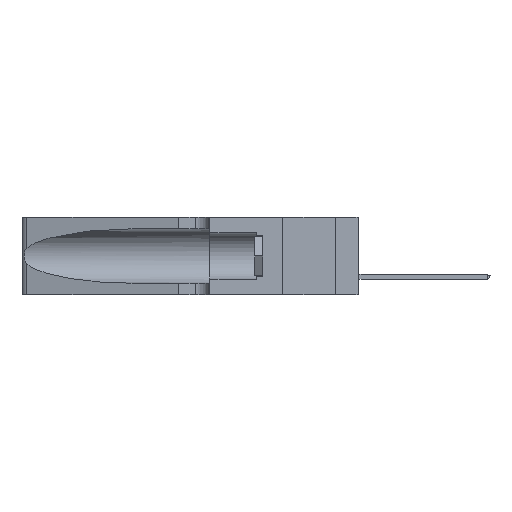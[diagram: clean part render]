
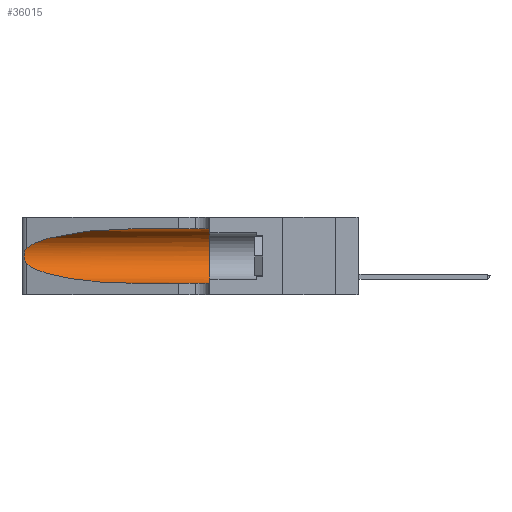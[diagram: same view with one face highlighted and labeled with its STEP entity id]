
A CAD part, left-side view. The second image highlights one B-rep face of the part: STEP entity #36015.
In plain terms, the highlighted cylindrical face has radius 3.308 mm (diameter 6.617 mm), a partial arc.
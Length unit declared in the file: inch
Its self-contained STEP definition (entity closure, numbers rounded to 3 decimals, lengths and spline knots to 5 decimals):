
#264 = CARTESIAN_POINT ( 'NONE',  ( 0.26075, 1.23896, 0.178 ) ) ;
#397 = CARTESIAN_POINT ( 'NONE',  ( 0.25487, 1.22718, 0.14631 ) ) ;
#412 = FACE_OUTER_BOUND ( 'NONE', #27075, .T. ) ;
#540 = CARTESIAN_POINT ( 'NONE',  ( 0.2373, 1.15595, 0.08982 ) ) ;
#809 = EDGE_CURVE ( 'NONE', #25328, #8005, #32476, .T. ) ;
#1909 = DIRECTION ( 'NONE',  ( 0., -1., 0. ) ) ;
#2008 = CYLINDRICAL_SURFACE ( 'NONE', #19978, 0.13025 ) ;
#3634 = CARTESIAN_POINT ( 'NONE',  ( 0.25789, 1.23486, 0.15765 ) ) ;
#3771 = CARTESIAN_POINT ( 'NONE',  ( 0.25555, 1.22993, 0.14849 ) ) ;
#4053 = CARTESIAN_POINT ( 'NONE',  ( 0.1305, 0.72297, 0.05475 ) ) ;
#4175 =( BOUNDED_CURVE ( )  B_SPLINE_CURVE ( 3, ( #26989, #540, #23588, #4053 ),
 .UNSPECIFIED., .F., .F. ) 
 B_SPLINE_CURVE_WITH_KNOTS ( ( 4, 4 ),
 ( 3.44316, 4.71239 ),
 .UNSPECIFIED. ) 
 CURVE ( )  GEOMETRIC_REPRESENTATION_ITEM ( )  RATIONAL_B_SPLINE_CURVE ( ( 1., 0.87, 0.87, 1. ) ) 
 REPRESENTATION_ITEM ( '' )  );
#4190 = CARTESIAN_POINT ( 'NONE',  ( 0.1305, 1.61858, 0.185 ) ) ;
#5490 = VERTEX_POINT ( 'NONE', #7061 ) ;
#6011 = ORIENTED_EDGE ( 'NONE', *, *, #38743, .T. ) ;
#6385 = EDGE_CURVE ( 'NONE', #8803, #22679, #4175, .T. ) ;
#6594 = EDGE_CURVE ( 'NONE', #8005, #26470, #9906, .T. ) ;
#7061 = CARTESIAN_POINT ( 'NONE',  ( 0.25487, 1.22718, 0.22369 ) ) ;
#7087 = CARTESIAN_POINT ( 'NONE',  ( 0.26075, 1.23896, 0.19203 ) ) ;
#8005 = VERTEX_POINT ( 'NONE', #24987 ) ;
#8803 = VERTEX_POINT ( 'NONE', #29382 ) ;
#9710 = ORIENTED_EDGE ( 'NONE', *, *, #809, .F. ) ;
#9906 = CIRCLE ( 'NONE', #33426, 0.13025 ) ;
#10192 = CARTESIAN_POINT ( 'NONE',  ( 0.25487, 1.22718, 0.22369 ) ) ;
#10298 = ORIENTED_EDGE ( 'NONE', *, *, #27484, .T. ) ;
#10596 = CARTESIAN_POINT ( 'NONE',  ( 0.26017, 1.23833, 0.17102 ) ) ;
#12334 = CARTESIAN_POINT ( 'NONE',  ( 0.18966, 0.96281, 0.31525 ) ) ;
#12624 = CARTESIAN_POINT ( 'NONE',  ( 0.25487, 1.22718, 0.22369 ) ) ;
#13598 = VECTOR ( 'NONE', #14438, 39.37008 ) ;
#13793 = CARTESIAN_POINT ( 'NONE',  ( 0.25555, 1.22994, 0.2215 ) ) ;
#13797 = DIRECTION ( 'NONE',  ( 0., -1., 0. ) ) ;
#14438 = DIRECTION ( 'NONE',  ( 0., -1., 0. ) ) ;
#15375 = LINE ( 'NONE', #21896, #42030 ) ;
#15705 = CARTESIAN_POINT ( 'NONE',  ( 0.2373, 1.15595, 0.28018 ) ) ;
#16502 = CARTESIAN_POINT ( 'NONE',  ( 0.1305, 0.72297, 0.05475 ) ) ;
#16868 = CARTESIAN_POINT ( 'NONE',  ( 0.26018, 1.23835, 0.19895 ) ) ;
#17226 =( BOUNDED_CURVE ( )  B_SPLINE_CURVE ( 3, ( #35673, #12334, #15705, #12624 ),
 .UNSPECIFIED., .F., .T. ) 
 B_SPLINE_CURVE_WITH_KNOTS ( ( 4, 4 ),
 ( 1.5708, 2.84003 ),
 .UNSPECIFIED. ) 
 CURVE ( )  GEOMETRIC_REPRESENTATION_ITEM ( )  RATIONAL_B_SPLINE_CURVE ( ( 1., 0.87, 0.87, 1. ) ) 
 REPRESENTATION_ITEM ( '' )  );
#17642 = CARTESIAN_POINT ( 'NONE',  ( 0.1305, 1.61858, 0.31525 ) ) ;
#19507 = ORIENTED_EDGE ( 'NONE', *, *, #6385, .T. ) ;
#19978 = AXIS2_PLACEMENT_3D ( 'NONE', #4190, #13797, #37297 ) ;
#21734 = DIRECTION ( 'NONE',  ( 0., 0., 1. ) ) ;
#21896 = CARTESIAN_POINT ( 'NONE',  ( 0.1305, 1.61858, 0.05475 ) ) ;
#22679 = VERTEX_POINT ( 'NONE', #16502 ) ;
#23378 = EDGE_CURVE ( 'NONE', #22679, #26470, #15375, .T. ) ;
#23588 = CARTESIAN_POINT ( 'NONE',  ( 0.18966, 0.96281, 0.05475 ) ) ;
#24987 = CARTESIAN_POINT ( 'NONE',  ( 0.1305, 0.35, 0.31525 ) ) ;
#25328 = VERTEX_POINT ( 'NONE', #25756 ) ;
#25348 = ORIENTED_EDGE ( 'NONE', *, *, #23378, .T. ) ;
#25756 = CARTESIAN_POINT ( 'NONE',  ( 0.1305, 0.72297, 0.31525 ) ) ;
#26470 = VERTEX_POINT ( 'NONE', #28781 ) ;
#26989 = CARTESIAN_POINT ( 'NONE',  ( 0.25487, 1.22718, 0.14631 ) ) ;
#27075 = EDGE_LOOP ( 'NONE', ( #6011, #10298, #19507, #25348, #29213, #9710 ) ) ;
#27132 = CARTESIAN_POINT ( 'NONE',  ( 0.25639, 1.23184, 0.21858 ) ) ;
#27484 = EDGE_CURVE ( 'NONE', #5490, #8803, #28827, .T. ) ;
#28288 = CARTESIAN_POINT ( 'NONE',  ( 0.1305, 0.35, 0.185 ) ) ;
#28781 = CARTESIAN_POINT ( 'NONE',  ( 0.1305, 0.35, 0.05475 ) ) ;
#28827 = B_SPLINE_CURVE_WITH_KNOTS ( 'NONE', 3,
 ( #10192, #13793, #27132, #37142, #30620, #16868, #7087, #264, #10596, #40218, #3634, #37000, #3771, #397 ),
 .UNSPECIFIED., .F., .F.,
 ( 4, 2, 2, 2, 2, 2, 4 ),
 ( 0., 0.00027, 0.00053, 0.00107, 0.0016, 0.00187, 0.00214 ),
 .UNSPECIFIED. ) ;
#29213 = ORIENTED_EDGE ( 'NONE', *, *, #6594, .F. ) ;
#29382 = CARTESIAN_POINT ( 'NONE',  ( 0.25487, 1.22718, 0.14631 ) ) ;
#30620 = CARTESIAN_POINT ( 'NONE',  ( 0.25854, 1.2359, 0.20912 ) ) ;
#32476 = LINE ( 'NONE', #17642, #13598 ) ;
#33426 = AXIS2_PLACEMENT_3D ( 'NONE', #28288, #41716, #21734 ) ;
#35673 = CARTESIAN_POINT ( 'NONE',  ( 0.1305, 0.72297, 0.31525 ) ) ;
#36015 = ADVANCED_FACE ( 'NONE', ( #412 ), #2008, .F. ) ;
#37000 = CARTESIAN_POINT ( 'NONE',  ( 0.25639, 1.23186, 0.15144 ) ) ;
#37142 = CARTESIAN_POINT ( 'NONE',  ( 0.25787, 1.23484, 0.2124 ) ) ;
#37297 = DIRECTION ( 'NONE',  ( 0., 0., -1. ) ) ;
#38743 = EDGE_CURVE ( 'NONE', #25328, #5490, #17226, .T. ) ;
#40218 = CARTESIAN_POINT ( 'NONE',  ( 0.25856, 1.23593, 0.16098 ) ) ;
#41716 = DIRECTION ( 'NONE',  ( 0., 1., 0. ) ) ;
#42030 = VECTOR ( 'NONE', #1909, 39.37008 ) ;
